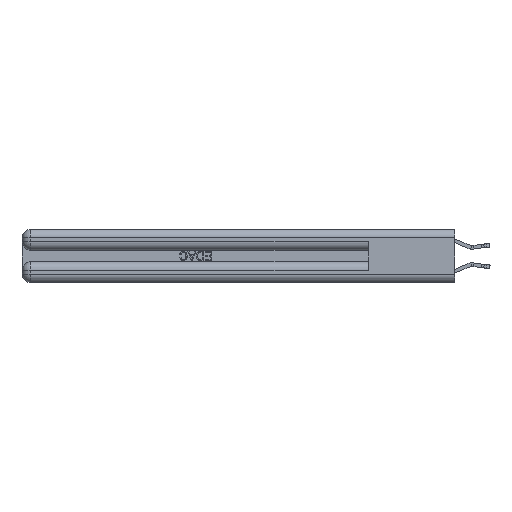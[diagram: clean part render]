
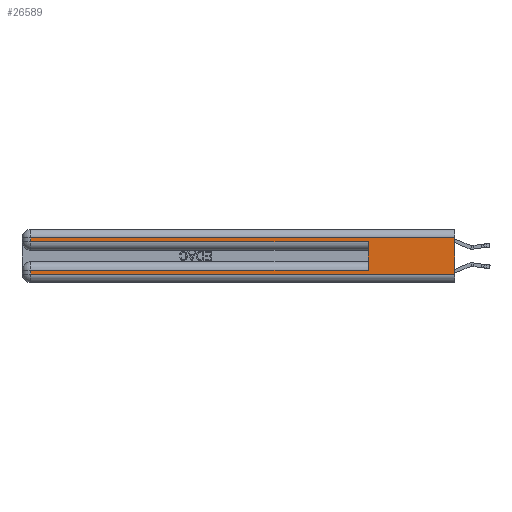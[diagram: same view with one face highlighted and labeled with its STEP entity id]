
A CAD part, left-side view. The second image highlights one B-rep face of the part: STEP entity #26589.
In plain terms, the highlighted planar face has unit normal (-1, 0, 0).
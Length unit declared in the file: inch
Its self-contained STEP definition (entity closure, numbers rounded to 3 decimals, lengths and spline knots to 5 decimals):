
#242 = VERTEX_POINT ( 'NONE', #11528 ) ;
#687 = VECTOR ( 'NONE', #22985, 39.37008 ) ;
#924 = VECTOR ( 'NONE', #1976, 39.37008 ) ;
#1185 = LINE ( 'NONE', #22241, #27831 ) ;
#1976 = DIRECTION ( 'NONE',  ( 0., -1., 0. ) ) ;
#2536 = CARTESIAN_POINT ( 'NONE',  ( 0., 0., 0.085 ) ) ;
#3060 = FACE_OUTER_BOUND ( 'NONE', #23900, .T. ) ;
#3733 = CARTESIAN_POINT ( 'NONE',  ( 0., 0.6, 0.285 ) ) ;
#4008 = CARTESIAN_POINT ( 'NONE',  ( 0., 0., 0.37 ) ) ;
#4169 = DIRECTION ( 'NONE',  ( 0., 1., 0. ) ) ;
#4202 = EDGE_CURVE ( 'NONE', #32560, #9250, #16820, .T. ) ;
#4411 = CARTESIAN_POINT ( 'NONE',  ( 0., 2.94, 0.37 ) ) ;
#5198 = VECTOR ( 'NONE', #4169, 39.37008 ) ;
#6811 = CARTESIAN_POINT ( 'NONE',  ( 0., 0., 0.31 ) ) ;
#7053 = DIRECTION ( 'NONE',  ( 0., 0., -1. ) ) ;
#7442 = CARTESIAN_POINT ( 'NONE',  ( 0., 2.94, 0.31 ) ) ;
#7681 = VECTOR ( 'NONE', #24953, 39.37008 ) ;
#8557 = EDGE_CURVE ( 'NONE', #32660, #22694, #25695, .T. ) ;
#8713 = EDGE_CURVE ( 'NONE', #242, #9364, #12214, .T. ) ;
#9250 = VERTEX_POINT ( 'NONE', #3733 ) ;
#9364 = VERTEX_POINT ( 'NONE', #22022 ) ;
#9422 = LINE ( 'NONE', #2536, #687 ) ;
#9439 = ORIENTED_EDGE ( 'NONE', *, *, #8713, .F. ) ;
#9533 = VERTEX_POINT ( 'NONE', #7442 ) ;
#11528 = CARTESIAN_POINT ( 'NONE',  ( 0., 0., 0.31 ) ) ;
#12117 = CARTESIAN_POINT ( 'NONE',  ( 0., 2.94, 0.285 ) ) ;
#12214 = LINE ( 'NONE', #4008, #30916 ) ;
#14270 = CARTESIAN_POINT ( 'NONE',  ( 0., 2.94, 0.37 ) ) ;
#14608 = EDGE_CURVE ( 'NONE', #16823, #9250, #22401, .T. ) ;
#15148 = LINE ( 'NONE', #6811, #5198 ) ;
#15497 = ORIENTED_EDGE ( 'NONE', *, *, #16239, .T. ) ;
#16239 = EDGE_CURVE ( 'NONE', #242, #9533, #15148, .T. ) ;
#16270 = ORIENTED_EDGE ( 'NONE', *, *, #30188, .T. ) ;
#16820 = LINE ( 'NONE', #27195, #924 ) ;
#16823 = VERTEX_POINT ( 'NONE', #24682 ) ;
#17337 = DIRECTION ( 'NONE',  ( 0., -1., 0. ) ) ;
#18732 = CARTESIAN_POINT ( 'NONE',  ( 0., 2.94, 0.06 ) ) ;
#18944 = VECTOR ( 'NONE', #21355, 39.37008 ) ;
#19258 = EDGE_CURVE ( 'NONE', #9533, #32560, #24531, .T. ) ;
#19715 = CARTESIAN_POINT ( 'NONE',  ( 0., 0.6, 0.145 ) ) ;
#19894 = ORIENTED_EDGE ( 'NONE', *, *, #14608, .F. ) ;
#21355 = DIRECTION ( 'NONE',  ( 0., 0., -1. ) ) ;
#22022 = CARTESIAN_POINT ( 'NONE',  ( 0., 0., 0.06 ) ) ;
#22183 = CARTESIAN_POINT ( 'NONE',  ( 0., 0., 0.37 ) ) ;
#22241 = CARTESIAN_POINT ( 'NONE',  ( 0., 0., 0.06 ) ) ;
#22401 = LINE ( 'NONE', #19715, #7681 ) ;
#22694 = VERTEX_POINT ( 'NONE', #18732 ) ;
#22985 = DIRECTION ( 'NONE',  ( 0., 1., 0. ) ) ;
#23722 = VECTOR ( 'NONE', #7053, 39.37008 ) ;
#23900 = EDGE_LOOP ( 'NONE', ( #9439, #15497, #30998, #31669, #19894, #28221, #27442, #16270 ) ) ;
#24531 = LINE ( 'NONE', #4411, #23722 ) ;
#24682 = CARTESIAN_POINT ( 'NONE',  ( 0., 0.6, 0.085 ) ) ;
#24953 = DIRECTION ( 'NONE',  ( 0., 0., 1. ) ) ;
#25084 = PLANE ( 'NONE',  #27917 ) ;
#25695 = LINE ( 'NONE', #14270, #18944 ) ;
#26589 = ADVANCED_FACE ( 'NONE', ( #3060 ), #25084, .F. ) ;
#26988 = DIRECTION ( 'NONE',  ( 0., 0., -1. ) ) ;
#27195 = CARTESIAN_POINT ( 'NONE',  ( 0., 0., 0.285 ) ) ;
#27442 = ORIENTED_EDGE ( 'NONE', *, *, #8557, .T. ) ;
#27533 = DIRECTION ( 'NONE',  ( 0., 0., -1. ) ) ;
#27831 = VECTOR ( 'NONE', #17337, 39.37008 ) ;
#27917 = AXIS2_PLACEMENT_3D ( 'NONE', #22183, #30217, #27533 ) ;
#28221 = ORIENTED_EDGE ( 'NONE', *, *, #31717, .T. ) ;
#30188 = EDGE_CURVE ( 'NONE', #22694, #9364, #1185, .T. ) ;
#30217 = DIRECTION ( 'NONE',  ( 1., 0., 0. ) ) ;
#30916 = VECTOR ( 'NONE', #26988, 39.37008 ) ;
#30998 = ORIENTED_EDGE ( 'NONE', *, *, #19258, .T. ) ;
#31669 = ORIENTED_EDGE ( 'NONE', *, *, #4202, .T. ) ;
#31717 = EDGE_CURVE ( 'NONE', #16823, #32660, #9422, .T. ) ;
#32560 = VERTEX_POINT ( 'NONE', #12117 ) ;
#32660 = VERTEX_POINT ( 'NONE', #32702 ) ;
#32702 = CARTESIAN_POINT ( 'NONE',  ( 0., 2.94, 0.085 ) ) ;
